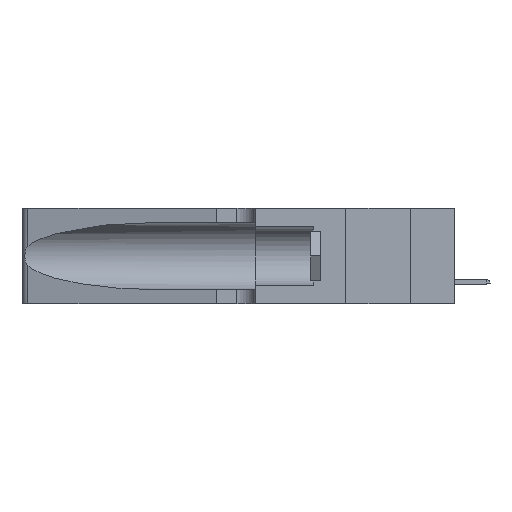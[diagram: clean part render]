
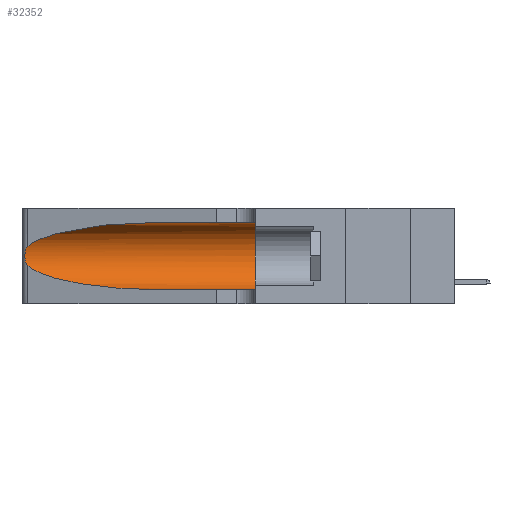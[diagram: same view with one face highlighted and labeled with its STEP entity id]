
A CAD part, left-side view. The second image highlights one B-rep face of the part: STEP entity #32352.
In plain terms, the highlighted cylindrical face has radius 3.308 mm (diameter 6.617 mm), a partial arc.
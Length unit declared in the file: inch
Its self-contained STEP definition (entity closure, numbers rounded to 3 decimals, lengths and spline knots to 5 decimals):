
#108 = CARTESIAN_POINT ( 'NONE',  ( 0.25789, 1.23486, 0.15765 ) ) ;
#143 = ORIENTED_EDGE ( 'NONE', *, *, #15077, .T. ) ;
#3083 = CARTESIAN_POINT ( 'NONE',  ( 0.25856, 1.23593, 0.16098 ) ) ;
#3294 = CARTESIAN_POINT ( 'NONE',  ( 0.25555, 1.22994, 0.2215 ) ) ;
#3453 = VERTEX_POINT ( 'NONE', #26166 ) ;
#4195 = ORIENTED_EDGE ( 'NONE', *, *, #41977, .T. ) ;
#6255 = CARTESIAN_POINT ( 'NONE',  ( 0.25787, 1.23484, 0.2124 ) ) ;
#6468 = CARTESIAN_POINT ( 'NONE',  ( 0.25555, 1.22993, 0.14849 ) ) ;
#6719 = CARTESIAN_POINT ( 'NONE',  ( 0.1305, 0.35, 0.05475 ) ) ;
#6976 = CARTESIAN_POINT ( 'NONE',  ( 0.1305, 0.72297, 0.31525 ) ) ;
#7187 = CARTESIAN_POINT ( 'NONE',  ( 0.18966, 0.96281, 0.05475 ) ) ;
#7400 = CARTESIAN_POINT ( 'NONE',  ( 0.25487, 1.22718, 0.22369 ) ) ;
#7455 = ORIENTED_EDGE ( 'NONE', *, *, #35392, .F. ) ;
#9195 = DIRECTION ( 'NONE',  ( 0., -1., 0. ) ) ;
#9894 = CARTESIAN_POINT ( 'NONE',  ( 0.26018, 1.23835, 0.19895 ) ) ;
#9965 = EDGE_CURVE ( 'NONE', #3453, #34098, #24297, .T. ) ;
#11457 = DIRECTION ( 'NONE',  ( 0., 1., 0. ) ) ;
#12092 = CARTESIAN_POINT ( 'NONE',  ( 0.1305, 0.35, 0.185 ) ) ;
#12517 = CARTESIAN_POINT ( 'NONE',  ( 0.25487, 1.22718, 0.14631 ) ) ;
#12541 = ORIENTED_EDGE ( 'NONE', *, *, #9965, .T. ) ;
#13316 = CARTESIAN_POINT ( 'NONE',  ( 0.25639, 1.23184, 0.21858 ) ) ;
#13844 = AXIS2_PLACEMENT_3D ( 'NONE', #12092, #11457, #28253 ) ;
#14032 = CARTESIAN_POINT ( 'NONE',  ( 0.2373, 1.15595, 0.28018 ) ) ;
#14523 = CIRCLE ( 'NONE', #13844, 0.13025 ) ;
#15077 = EDGE_CURVE ( 'NONE', #31463, #24099, #30473, .T. ) ;
#15313 = VECTOR ( 'NONE', #37696, 39.37008 ) ;
#16619 = EDGE_CURVE ( 'NONE', #3453, #24905, #28746, .T. ) ;
#16919 = CARTESIAN_POINT ( 'NONE',  ( 0.25487, 1.22718, 0.14631 ) ) ;
#18471 = B_SPLINE_CURVE_WITH_KNOTS ( 'NONE', 3,
 ( #38594, #3294, #13316, #6255, #32236, #9894, #35620, #36250, #22886, #3083, #108, #23082, #6468, #16919 ),
 .UNSPECIFIED., .F., .F.,
 ( 4, 2, 2, 2, 2, 2, 4 ),
 ( 0., 0.00027, 0.00053, 0.00107, 0.0016, 0.00187, 0.00214 ),
 .UNSPECIFIED. ) ;
#18604 = CYLINDRICAL_SURFACE ( 'NONE', #38093, 0.13025 ) ;
#19764 = CARTESIAN_POINT ( 'NONE',  ( 0.1305, 0.72297, 0.05475 ) ) ;
#20112 = VECTOR ( 'NONE', #9195, 39.37008 ) ;
#22886 = CARTESIAN_POINT ( 'NONE',  ( 0.26017, 1.23833, 0.17102 ) ) ;
#22952 = CARTESIAN_POINT ( 'NONE',  ( 0.25487, 1.22718, 0.14631 ) ) ;
#23082 = CARTESIAN_POINT ( 'NONE',  ( 0.25639, 1.23186, 0.15144 ) ) ;
#23442 = CARTESIAN_POINT ( 'NONE',  ( 0.1305, 0.35, 0.31525 ) ) ;
#24099 = VERTEX_POINT ( 'NONE', #6719 ) ;
#24297 =( BOUNDED_CURVE ( )  B_SPLINE_CURVE ( 3, ( #6976, #36541, #14032, #7400 ),
 .UNSPECIFIED., .F., .T. ) 
 B_SPLINE_CURVE_WITH_KNOTS ( ( 4, 4 ),
 ( 1.5708, 2.84003 ),
 .UNSPECIFIED. ) 
 CURVE ( )  GEOMETRIC_REPRESENTATION_ITEM ( )  RATIONAL_B_SPLINE_CURVE ( ( 1., 0.87, 0.87, 1. ) ) 
 REPRESENTATION_ITEM ( '' )  );
#24905 = VERTEX_POINT ( 'NONE', #23442 ) ;
#25578 = EDGE_LOOP ( 'NONE', ( #12541, #33430, #4195, #143, #7455, #29389 ) ) ;
#26166 = CARTESIAN_POINT ( 'NONE',  ( 0.1305, 0.72297, 0.31525 ) ) ;
#27537 = CARTESIAN_POINT ( 'NONE',  ( 0.1305, 1.61858, 0.185 ) ) ;
#28253 = DIRECTION ( 'NONE',  ( 0., 0., 1. ) ) ;
#28376 = DIRECTION ( 'NONE',  ( 0., 0., -1. ) ) ;
#28746 = LINE ( 'NONE', #38312, #20112 ) ;
#29389 = ORIENTED_EDGE ( 'NONE', *, *, #16619, .F. ) ;
#29436 = VERTEX_POINT ( 'NONE', #12517 ) ;
#30473 = LINE ( 'NONE', #40457, #15313 ) ;
#31109 = CARTESIAN_POINT ( 'NONE',  ( 0.25487, 1.22718, 0.22369 ) ) ;
#31463 = VERTEX_POINT ( 'NONE', #37448 ) ;
#32236 = CARTESIAN_POINT ( 'NONE',  ( 0.25854, 1.2359, 0.20912 ) ) ;
#32352 = ADVANCED_FACE ( 'NONE', ( #34324 ), #18604, .F. ) ;
#33430 = ORIENTED_EDGE ( 'NONE', *, *, #39091, .T. ) ;
#34098 = VERTEX_POINT ( 'NONE', #31109 ) ;
#34103 = DIRECTION ( 'NONE',  ( 0., -1., 0. ) ) ;
#34324 = FACE_OUTER_BOUND ( 'NONE', #25578, .T. ) ;
#35392 = EDGE_CURVE ( 'NONE', #24905, #24099, #14523, .T. ) ;
#35620 = CARTESIAN_POINT ( 'NONE',  ( 0.26075, 1.23896, 0.19203 ) ) ;
#35907 = CARTESIAN_POINT ( 'NONE',  ( 0.2373, 1.15595, 0.08982 ) ) ;
#36250 = CARTESIAN_POINT ( 'NONE',  ( 0.26075, 1.23896, 0.178 ) ) ;
#36541 = CARTESIAN_POINT ( 'NONE',  ( 0.18966, 0.96281, 0.31525 ) ) ;
#37448 = CARTESIAN_POINT ( 'NONE',  ( 0.1305, 0.72297, 0.05475 ) ) ;
#37696 = DIRECTION ( 'NONE',  ( 0., -1., 0. ) ) ;
#38093 = AXIS2_PLACEMENT_3D ( 'NONE', #27537, #34103, #28376 ) ;
#38312 = CARTESIAN_POINT ( 'NONE',  ( 0.1305, 1.61858, 0.31525 ) ) ;
#38594 = CARTESIAN_POINT ( 'NONE',  ( 0.25487, 1.22718, 0.22369 ) ) ;
#39091 = EDGE_CURVE ( 'NONE', #34098, #29436, #18471, .T. ) ;
#40457 = CARTESIAN_POINT ( 'NONE',  ( 0.1305, 1.61858, 0.05475 ) ) ;
#41655 =( BOUNDED_CURVE ( )  B_SPLINE_CURVE ( 3, ( #22952, #35907, #7187, #19764 ),
 .UNSPECIFIED., .F., .T. ) 
 B_SPLINE_CURVE_WITH_KNOTS ( ( 4, 4 ),
 ( 3.44316, 4.71239 ),
 .UNSPECIFIED. ) 
 CURVE ( )  GEOMETRIC_REPRESENTATION_ITEM ( )  RATIONAL_B_SPLINE_CURVE ( ( 1., 0.87, 0.87, 1. ) ) 
 REPRESENTATION_ITEM ( '' )  );
#41977 = EDGE_CURVE ( 'NONE', #29436, #31463, #41655, .T. ) ;
